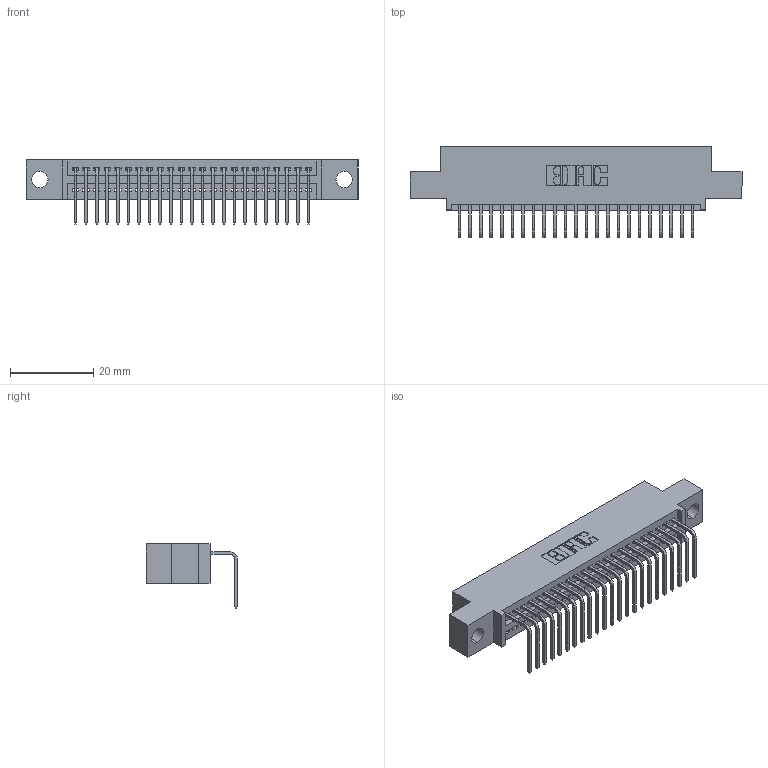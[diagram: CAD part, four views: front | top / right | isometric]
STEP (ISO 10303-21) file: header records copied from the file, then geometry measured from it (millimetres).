
FILE_DESCRIPTION (( 'STEP AP203' ), '1' );
FILE_NAME ('395-023-558-404.STEP', '2021-06-11T14:19:07', ( '' ), ( '' ), 'SwSTEP 2.0', 'SolidWorks 2020', '' );
FILE_SCHEMA (( 'CONFIG_CONTROL_DESIGN' ));
Length unit declared in the file: inch
Products named in the file (3): 345 Part_0.110 Offset - 0.156 Dia-TI; 395-023-558-404; 345-292-001_558 Tail - 2
Assembly tree (24 placements, depth 2):
  395-023-558-404
    345 Part_0.110 Offset - 0.156 Dia-TI
    345-292-001_558 Tail - 2  x23
Bounding box: 79.63 x 21.83 x 15.37 mm (x, y, z)
Volume: 7304.9 mm3; surface area: 9824 mm2
Topology: 24 solids, 24 shells, 1524 faces, 4575 edges, 3018 vertices
Faces by surface type: plane 1064, cylinder 460
Entity records: 20503 total; most frequent: CARTESIAN_POINT 3563, ORIENTED_EDGE 3518, DIRECTION 3137, EDGE_CURVE 1759, LINE 1535, VECTOR 1535, VERTEX_POINT 1170, AXIS2_PLACEMENT_3D 801
